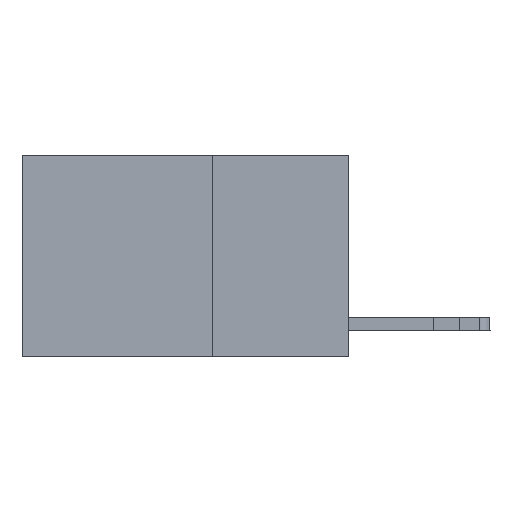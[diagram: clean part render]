
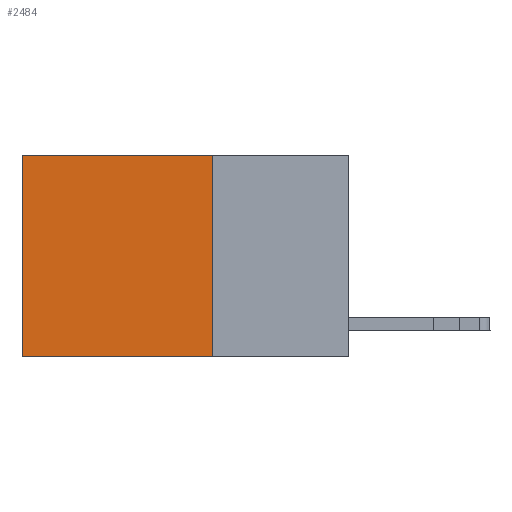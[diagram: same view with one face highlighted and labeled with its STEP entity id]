
A CAD part, left-side view. The second image highlights one B-rep face of the part: STEP entity #2484.
In plain terms, the highlighted planar face has unit normal (-1, 0, 0).
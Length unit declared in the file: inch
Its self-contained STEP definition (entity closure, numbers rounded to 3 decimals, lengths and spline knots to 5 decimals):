
#1231 = CARTESIAN_POINT ( 'NONE',  ( 0.2625, 0.25, 0. ) ) ;
#1325 = DIRECTION ( 'NONE',  ( 0., 0., -1. ) ) ;
#2484 = ADVANCED_FACE ( 'NONE', ( #5276 ), #19028, .F. ) ;
#2740 = VERTEX_POINT ( 'NONE', #21409 ) ;
#2962 = DIRECTION ( 'NONE',  ( 1., 0., 0. ) ) ;
#4566 = AXIS2_PLACEMENT_3D ( 'NONE', #1231, #2962, #7771 ) ;
#5276 = FACE_OUTER_BOUND ( 'NONE', #18500, .T. ) ;
#5620 = EDGE_CURVE ( 'NONE', #8322, #2740, #18002, .T. ) ;
#7137 = VERTEX_POINT ( 'NONE', #16687 ) ;
#7413 = CARTESIAN_POINT ( 'NONE',  ( 0.2625, 0.25, 0. ) ) ;
#7606 = LINE ( 'NONE', #9146, #16691 ) ;
#7661 = VERTEX_POINT ( 'NONE', #10432 ) ;
#7771 = DIRECTION ( 'NONE',  ( 0., 0., -1. ) ) ;
#7951 = DIRECTION ( 'NONE',  ( 0., 0., -1. ) ) ;
#8322 = VERTEX_POINT ( 'NONE', #11469 ) ;
#9146 = CARTESIAN_POINT ( 'NONE',  ( 0.2625, 0.25, -0.37 ) ) ;
#9160 = LINE ( 'NONE', #7413, #15633 ) ;
#9938 = VECTOR ( 'NONE', #7951, 39.37008 ) ;
#10432 = CARTESIAN_POINT ( 'NONE',  ( 0.2625, 0.25, -0.37 ) ) ;
#10483 = ORIENTED_EDGE ( 'NONE', *, *, #5620, .T. ) ;
#11469 = CARTESIAN_POINT ( 'NONE',  ( 0.2625, 0.6, 0. ) ) ;
#11662 = CARTESIAN_POINT ( 'NONE',  ( 0.2625, 0.25, 0. ) ) ;
#12301 = DIRECTION ( 'NONE',  ( 0., 1., 0. ) ) ;
#12356 = EDGE_CURVE ( 'NONE', #7661, #2740, #7606, .T. ) ;
#12743 = CARTESIAN_POINT ( 'NONE',  ( 0.2625, 0.6, 0. ) ) ;
#13040 = ORIENTED_EDGE ( 'NONE', *, *, #12356, .F. ) ;
#14821 = LINE ( 'NONE', #11662, #15571 ) ;
#14963 = EDGE_CURVE ( 'NONE', #7137, #7661, #14821, .T. ) ;
#15571 = VECTOR ( 'NONE', #1325, 39.37008 ) ;
#15633 = VECTOR ( 'NONE', #15912, 39.37008 ) ;
#15912 = DIRECTION ( 'NONE',  ( 0., 1., 0. ) ) ;
#16597 = EDGE_CURVE ( 'NONE', #7137, #8322, #9160, .T. ) ;
#16687 = CARTESIAN_POINT ( 'NONE',  ( 0.2625, 0.25, 0. ) ) ;
#16691 = VECTOR ( 'NONE', #12301, 39.37008 ) ;
#18002 = LINE ( 'NONE', #12743, #9938 ) ;
#18500 = EDGE_LOOP ( 'NONE', ( #10483, #13040, #19601, #19727 ) ) ;
#19028 = PLANE ( 'NONE',  #4566 ) ;
#19601 = ORIENTED_EDGE ( 'NONE', *, *, #14963, .F. ) ;
#19727 = ORIENTED_EDGE ( 'NONE', *, *, #16597, .T. ) ;
#21409 = CARTESIAN_POINT ( 'NONE',  ( 0.2625, 0.6, -0.37 ) ) ;
